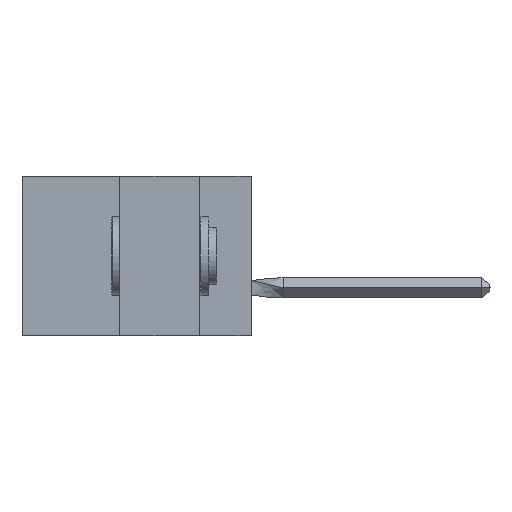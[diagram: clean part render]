
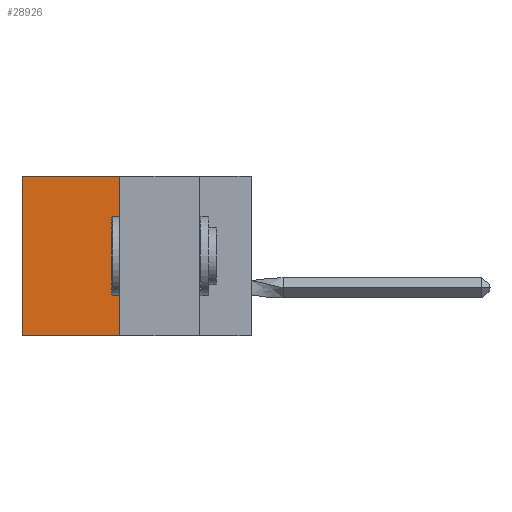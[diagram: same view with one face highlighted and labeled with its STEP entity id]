
A CAD part, left-side view. The second image highlights one B-rep face of the part: STEP entity #28926.
In plain terms, the highlighted planar face has unit normal (-1, 0, 0).
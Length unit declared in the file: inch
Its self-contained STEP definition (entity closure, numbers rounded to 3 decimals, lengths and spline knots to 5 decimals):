
#500 = DIRECTION ( 'NONE',  ( 0., 0., -1. ) ) ;
#925 = LINE ( 'NONE', #32009, #22570 ) ;
#4665 = CARTESIAN_POINT ( 'NONE',  ( 0.305, 0.413, -0.5 ) ) ;
#6599 = DIRECTION ( 'NONE',  ( 0., 0., -1. ) ) ;
#8256 = DIRECTION ( 'NONE',  ( 0., 1., 0. ) ) ;
#11201 = CARTESIAN_POINT ( 'NONE',  ( 0.305, 0.413, -0.5 ) ) ;
#11915 = ORIENTED_EDGE ( 'NONE', *, *, #18970, .F. ) ;
#12311 = CARTESIAN_POINT ( 'NONE',  ( 0.305, 0.72, -0.5 ) ) ;
#12682 = CARTESIAN_POINT ( 'NONE',  ( 0.305, 0.413, -0.5 ) ) ;
#14079 = CARTESIAN_POINT ( 'NONE',  ( 0.305, 0.413, -0.5 ) ) ;
#14912 = VERTEX_POINT ( 'NONE', #12311 ) ;
#15106 = EDGE_CURVE ( 'NONE', #19752, #14912, #925, .T. ) ;
#16938 = CARTESIAN_POINT ( 'NONE',  ( 0.305, 0.413, 0. ) ) ;
#18206 = ORIENTED_EDGE ( 'NONE', *, *, #19642, .T. ) ;
#18728 = VECTOR ( 'NONE', #21659, 39.37008 ) ;
#18966 = ORIENTED_EDGE ( 'NONE', *, *, #15106, .T. ) ;
#18970 = EDGE_CURVE ( 'NONE', #22220, #24273, #28170, .T. ) ;
#19642 = EDGE_CURVE ( 'NONE', #22220, #19752, #19972, .T. ) ;
#19752 = VERTEX_POINT ( 'NONE', #34687 ) ;
#19972 = LINE ( 'NONE', #16938, #32639 ) ;
#21659 = DIRECTION ( 'NONE',  ( 0., 0., -1. ) ) ;
#22220 = VERTEX_POINT ( 'NONE', #25132 ) ;
#22570 = VECTOR ( 'NONE', #500, 39.37008 ) ;
#24273 = VERTEX_POINT ( 'NONE', #11201 ) ;
#24950 = EDGE_LOOP ( 'NONE', ( #18966, #26199, #11915, #18206 ) ) ;
#25132 = CARTESIAN_POINT ( 'NONE',  ( 0.305, 0.413, 0. ) ) ;
#26199 = ORIENTED_EDGE ( 'NONE', *, *, #26783, .F. ) ;
#26783 = EDGE_CURVE ( 'NONE', #24273, #14912, #27086, .T. ) ;
#27086 = LINE ( 'NONE', #14079, #33388 ) ;
#28170 = LINE ( 'NONE', #4665, #18728 ) ;
#28926 = ADVANCED_FACE ( 'NONE', ( #35084 ), #32681, .F. ) ;
#32009 = CARTESIAN_POINT ( 'NONE',  ( 0.305, 0.72, -0.5 ) ) ;
#32296 = DIRECTION ( 'NONE',  ( 1., 0., 0. ) ) ;
#32639 = VECTOR ( 'NONE', #34429, 39.37008 ) ;
#32681 = PLANE ( 'NONE',  #33890 ) ;
#33388 = VECTOR ( 'NONE', #8256, 39.37008 ) ;
#33890 = AXIS2_PLACEMENT_3D ( 'NONE', #12682, #32296, #6599 ) ;
#34429 = DIRECTION ( 'NONE',  ( 0., 1., 0. ) ) ;
#34687 = CARTESIAN_POINT ( 'NONE',  ( 0.305, 0.72, 0. ) ) ;
#35084 = FACE_OUTER_BOUND ( 'NONE', #24950, .T. ) ;
